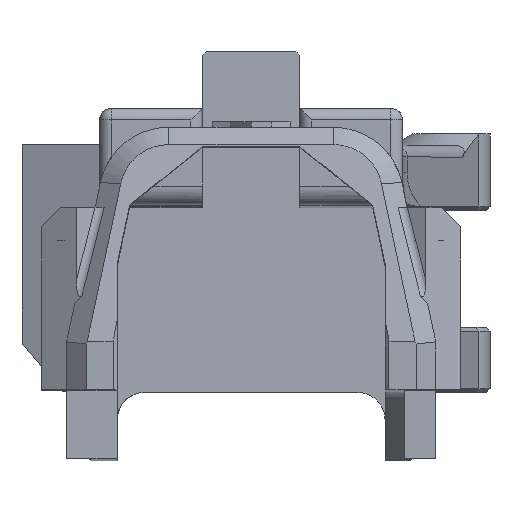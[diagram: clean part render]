
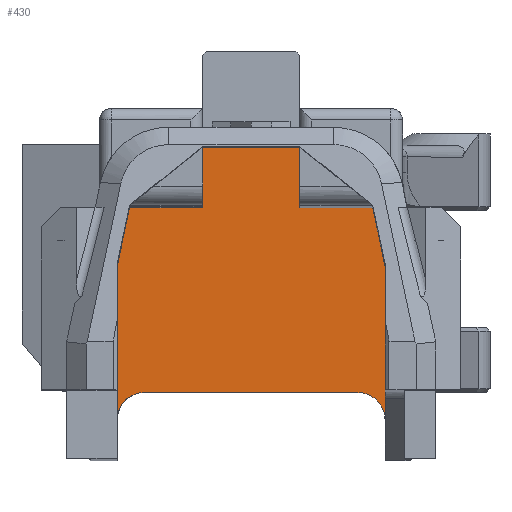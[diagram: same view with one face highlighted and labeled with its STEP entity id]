
A CAD part, top view. The second image highlights one B-rep face of the part: STEP entity #430.
In plain terms, the highlighted planar face has unit normal (0, 0, 1).
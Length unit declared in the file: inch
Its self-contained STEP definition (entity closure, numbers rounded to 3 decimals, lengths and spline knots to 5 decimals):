
#19 = CARTESIAN_POINT ( 'NONE',  ( 0.68898, 0.65, -8.38 ) ) ;
#138 = EDGE_CURVE ( 'NONE', #4622, #1395, #10549, .T. ) ;
#179 = EDGE_CURVE ( 'NONE', #3302, #9629, #13258, .T. ) ;
#430 = ADVANCED_FACE ( 'NONE', ( #4962 ), #7166, .F. ) ;
#711 = DIRECTION ( 'NONE',  ( 0., -1., 0. ) ) ;
#997 = CARTESIAN_POINT ( 'NONE',  ( 0.25, 0.95, -8.38 ) ) ;
#1069 = ORIENTED_EDGE ( 'NONE', *, *, #11168, .F. ) ;
#1071 = LINE ( 'NONE', #4159, #9884 ) ;
#1072 = ORIENTED_EDGE ( 'NONE', *, *, #2855, .F. ) ;
#1370 = LINE ( 'NONE', #11673, #7078 ) ;
#1395 = VERTEX_POINT ( 'NONE', #19 ) ;
#1413 = LINE ( 'NONE', #12748, #4608 ) ;
#1423 = AXIS2_PLACEMENT_3D ( 'NONE', #8565, #5128, #7473 ) ;
#1484 = CARTESIAN_POINT ( 'NONE',  ( -0.68898, 0., -8.38 ) ) ;
#1500 = ORIENTED_EDGE ( 'NONE', *, *, #4104, .T. ) ;
#1572 = ORIENTED_EDGE ( 'NONE', *, *, #2632, .T. ) ;
#1599 = VECTOR ( 'NONE', #7031, 39.37008 ) ;
#1863 = CARTESIAN_POINT ( 'NONE',  ( 0.69882, -1.4, -8.38 ) ) ;
#1928 = DIRECTION ( 'NONE',  ( 0., 0., -1. ) ) ;
#1943 = CARTESIAN_POINT ( 'NONE',  ( 0.25, 0., -8.38 ) ) ;
#2097 = DIRECTION ( 'NONE',  ( 1., 0., 0. ) ) ;
#2156 = CARTESIAN_POINT ( 'NONE',  ( 0.62521, 0.95, -8.38 ) ) ;
#2467 = EDGE_CURVE ( 'NONE', #9447, #8546, #4998, .T. ) ;
#2518 = LINE ( 'NONE', #1484, #11419 ) ;
#2632 = EDGE_CURVE ( 'NONE', #10074, #11075, #1071, .T. ) ;
#2686 = EDGE_CURVE ( 'NONE', #4622, #6420, #12496, .T. ) ;
#2708 = LINE ( 'NONE', #5731, #3859 ) ;
#2808 = ORIENTED_EDGE ( 'NONE', *, *, #179, .F. ) ;
#2855 = EDGE_CURVE ( 'NONE', #6420, #3302, #1413, .T. ) ;
#3096 = LINE ( 'NONE', #7310, #1599 ) ;
#3107 = VERTEX_POINT ( 'NONE', #12017 ) ;
#3125 = DIRECTION ( 'NONE',  ( -1., 0., 0. ) ) ;
#3173 = VERTEX_POINT ( 'NONE', #12081 ) ;
#3228 = ORIENTED_EDGE ( 'NONE', *, *, #6457, .F. ) ;
#3302 = VERTEX_POINT ( 'NONE', #8112 ) ;
#3379 = CARTESIAN_POINT ( 'NONE',  ( 0.38, 1.31, -8.38 ) ) ;
#3764 = VECTOR ( 'NONE', #11348, 39.37008 ) ;
#3859 = VECTOR ( 'NONE', #711, 39.37008 ) ;
#3869 = EDGE_CURVE ( 'NONE', #8546, #9629, #2518, .T. ) ;
#4007 = VECTOR ( 'NONE', #6369, 39.37008 ) ;
#4104 = EDGE_CURVE ( 'NONE', #3107, #3173, #9724, .T. ) ;
#4138 = CARTESIAN_POINT ( 'NONE',  ( -0.38, 1.31, -8.38 ) ) ;
#4155 = CARTESIAN_POINT ( 'NONE',  ( 0.68898, 0.65, -8.38 ) ) ;
#4159 = CARTESIAN_POINT ( 'NONE',  ( 0.38, 1.31, -8.38 ) ) ;
#4312 = LINE ( 'NONE', #12408, #4007 ) ;
#4431 = VECTOR ( 'NONE', #13458, 39.37008 ) ;
#4608 = VECTOR ( 'NONE', #11847, 39.37008 ) ;
#4622 = VERTEX_POINT ( 'NONE', #13363 ) ;
#4694 = ORIENTED_EDGE ( 'NONE', *, *, #6181, .T. ) ;
#4962 = FACE_OUTER_BOUND ( 'NONE', #12550, .T. ) ;
#4998 = LINE ( 'NONE', #6929, #9005 ) ;
#5128 = DIRECTION ( 'NONE',  ( 0., 0., 1. ) ) ;
#5301 = VERTEX_POINT ( 'NONE', #7770 ) ;
#5392 = VECTOR ( 'NONE', #6137, 39.37008 ) ;
#5525 = VERTEX_POINT ( 'NONE', #8300 ) ;
#5567 = DIRECTION ( 'NONE',  ( 1., 0., 0. ) ) ;
#5731 = CARTESIAN_POINT ( 'NONE',  ( -0.38, 1.05, -8.38 ) ) ;
#5911 = CARTESIAN_POINT ( 'NONE',  ( -0.25, 0., -8.38 ) ) ;
#5916 = AXIS2_PLACEMENT_3D ( 'NONE', #7412, #8358, #2097 ) ;
#6063 = LINE ( 'NONE', #13332, #3764 ) ;
#6087 = ORIENTED_EDGE ( 'NONE', *, *, #8225, .T. ) ;
#6137 = DIRECTION ( 'NONE',  ( 0., -1., 0. ) ) ;
#6181 = EDGE_CURVE ( 'NONE', #3173, #10074, #3096, .T. ) ;
#6215 = EDGE_CURVE ( 'NONE', #11068, #13080, #6063, .T. ) ;
#6369 = DIRECTION ( 'NONE',  ( -1., 0., 0. ) ) ;
#6420 = VERTEX_POINT ( 'NONE', #8814 ) ;
#6457 = EDGE_CURVE ( 'NONE', #7428, #5525, #9287, .T. ) ;
#6880 = ORIENTED_EDGE ( 'NONE', *, *, #6215, .T. ) ;
#6929 = CARTESIAN_POINT ( 'NONE',  ( -0.68898, 0.65, -8.38 ) ) ;
#7031 = DIRECTION ( 'NONE',  ( 0., 1., 0. ) ) ;
#7078 = VECTOR ( 'NONE', #5567, 39.37008 ) ;
#7166 = PLANE ( 'NONE',  #8029 ) ;
#7174 = CARTESIAN_POINT ( 'NONE',  ( -0.68898, 0.65, -8.38 ) ) ;
#7265 = ORIENTED_EDGE ( 'NONE', *, *, #7690, .T. ) ;
#7310 = CARTESIAN_POINT ( 'NONE',  ( 0.38, 1.05, -8.38 ) ) ;
#7412 = CARTESIAN_POINT ( 'NONE',  ( 0.54898, -0.14, -8.38 ) ) ;
#7428 = VERTEX_POINT ( 'NONE', #7923 ) ;
#7473 = DIRECTION ( 'NONE',  ( -1., 0., 0. ) ) ;
#7579 = ORIENTED_EDGE ( 'NONE', *, *, #9738, .T. ) ;
#7690 = EDGE_CURVE ( 'NONE', #5301, #5525, #1370, .T. ) ;
#7730 = CARTESIAN_POINT ( 'NONE',  ( 0.25, 1.05, -8.38 ) ) ;
#7770 = CARTESIAN_POINT ( 'NONE',  ( -0.38, 1.05, -8.38 ) ) ;
#7923 = CARTESIAN_POINT ( 'NONE',  ( -0.25, 0.95, -8.38 ) ) ;
#8029 = AXIS2_PLACEMENT_3D ( 'NONE', #1863, #1928, #13465 ) ;
#8112 = CARTESIAN_POINT ( 'NONE',  ( -0.54898, 0., -8.38 ) ) ;
#8225 = EDGE_CURVE ( 'NONE', #7428, #9447, #4312, .T. ) ;
#8300 = CARTESIAN_POINT ( 'NONE',  ( -0.25, 1.05, -8.38 ) ) ;
#8358 = DIRECTION ( 'NONE',  ( 0., 0., 1. ) ) ;
#8546 = VERTEX_POINT ( 'NONE', #7174 ) ;
#8565 = CARTESIAN_POINT ( 'NONE',  ( -0.54898, -0.14, -8.38 ) ) ;
#8814 = CARTESIAN_POINT ( 'NONE',  ( 0.54898, 0., -8.38 ) ) ;
#8848 = DIRECTION ( 'NONE',  ( 0., -1., 0. ) ) ;
#9005 = VECTOR ( 'NONE', #11307, 39.37008 ) ;
#9287 = LINE ( 'NONE', #5911, #4431 ) ;
#9308 = VECTOR ( 'NONE', #10421, 39.37008 ) ;
#9447 = VERTEX_POINT ( 'NONE', #9820 ) ;
#9456 = LINE ( 'NONE', #2156, #13034 ) ;
#9629 = VERTEX_POINT ( 'NONE', #11031 ) ;
#9724 = LINE ( 'NONE', #7730, #12298 ) ;
#9738 = EDGE_CURVE ( 'NONE', #1395, #11068, #9456, .T. ) ;
#9785 = ORIENTED_EDGE ( 'NONE', *, *, #138, .T. ) ;
#9820 = CARTESIAN_POINT ( 'NONE',  ( -0.62521, 0.95, -8.38 ) ) ;
#9884 = VECTOR ( 'NONE', #3125, 39.37008 ) ;
#10074 = VERTEX_POINT ( 'NONE', #3379 ) ;
#10421 = DIRECTION ( 'NONE',  ( 0., 1., 0. ) ) ;
#10481 = DIRECTION ( 'NONE',  ( -0.208, 0.978, 0. ) ) ;
#10521 = ORIENTED_EDGE ( 'NONE', *, *, #2467, .T. ) ;
#10549 = LINE ( 'NONE', #4155, #9308 ) ;
#10875 = DIRECTION ( 'NONE',  ( 1., 0., 0. ) ) ;
#11031 = CARTESIAN_POINT ( 'NONE',  ( -0.68898, -0.14, -8.38 ) ) ;
#11068 = VERTEX_POINT ( 'NONE', #11483 ) ;
#11075 = VERTEX_POINT ( 'NONE', #4138 ) ;
#11168 = EDGE_CURVE ( 'NONE', #3107, #13080, #11353, .T. ) ;
#11252 = ORIENTED_EDGE ( 'NONE', *, *, #2686, .F. ) ;
#11307 = DIRECTION ( 'NONE',  ( -0.208, -0.978, 0. ) ) ;
#11348 = DIRECTION ( 'NONE',  ( -1., 0., 0. ) ) ;
#11353 = LINE ( 'NONE', #1943, #5392 ) ;
#11419 = VECTOR ( 'NONE', #8848, 39.37008 ) ;
#11483 = CARTESIAN_POINT ( 'NONE',  ( 0.62521, 0.95, -8.38 ) ) ;
#11673 = CARTESIAN_POINT ( 'NONE',  ( -0.25, 1.05, -8.38 ) ) ;
#11847 = DIRECTION ( 'NONE',  ( -1., 0., 0. ) ) ;
#12017 = CARTESIAN_POINT ( 'NONE',  ( 0.25, 1.05, -8.38 ) ) ;
#12081 = CARTESIAN_POINT ( 'NONE',  ( 0.38, 1.05, -8.38 ) ) ;
#12298 = VECTOR ( 'NONE', #10875, 39.37008 ) ;
#12408 = CARTESIAN_POINT ( 'NONE',  ( -0.62521, 0.95, -8.38 ) ) ;
#12496 = CIRCLE ( 'NONE', #5916, 0.14 ) ;
#12550 = EDGE_LOOP ( 'NONE', ( #12795, #2808, #1072, #11252, #9785, #7579, #6880, #1069, #1500, #4694, #1572, #13032, #7265, #3228, #6087, #10521 ) ) ;
#12748 = CARTESIAN_POINT ( 'NONE',  ( -0.54898, 0., -8.38 ) ) ;
#12795 = ORIENTED_EDGE ( 'NONE', *, *, #3869, .T. ) ;
#13032 = ORIENTED_EDGE ( 'NONE', *, *, #13400, .T. ) ;
#13034 = VECTOR ( 'NONE', #10481, 39.37008 ) ;
#13080 = VERTEX_POINT ( 'NONE', #997 ) ;
#13258 = CIRCLE ( 'NONE', #1423, 0.14 ) ;
#13332 = CARTESIAN_POINT ( 'NONE',  ( -0.62521, 0.95, -8.38 ) ) ;
#13363 = CARTESIAN_POINT ( 'NONE',  ( 0.68898, -0.14, -8.38 ) ) ;
#13400 = EDGE_CURVE ( 'NONE', #11075, #5301, #2708, .T. ) ;
#13458 = DIRECTION ( 'NONE',  ( 0., 1., 0. ) ) ;
#13465 = DIRECTION ( 'NONE',  ( -1., 0., 0. ) ) ;
